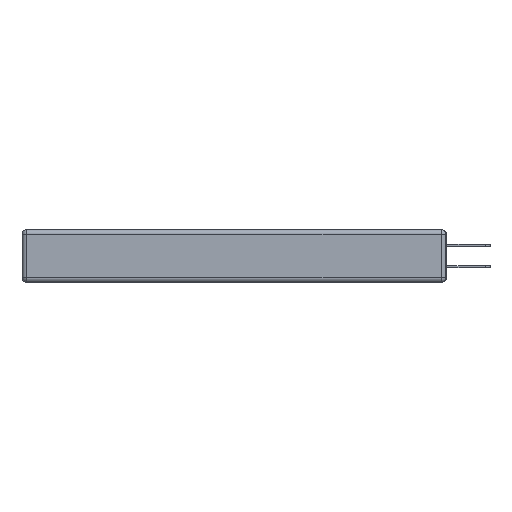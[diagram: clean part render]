
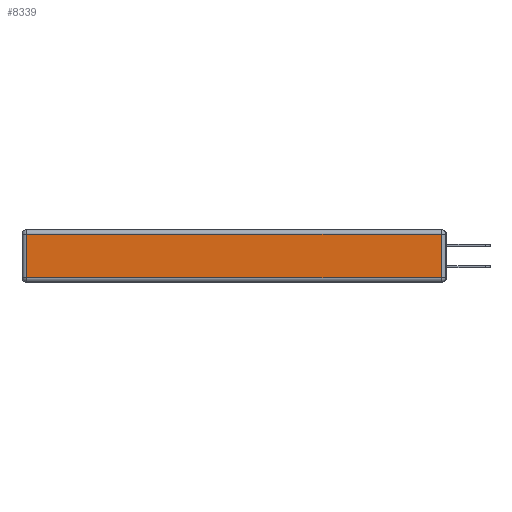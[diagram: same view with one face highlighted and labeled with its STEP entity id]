
A CAD part, left-side view. The second image highlights one B-rep face of the part: STEP entity #8339.
In plain terms, the highlighted planar face has unit normal (-1, 0, 0).
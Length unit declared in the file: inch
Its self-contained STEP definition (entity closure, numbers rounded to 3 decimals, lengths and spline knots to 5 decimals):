
#351 = LINE ( 'NONE', #5367, #19564 ) ;
#704 = LINE ( 'NONE', #6804, #16966 ) ;
#1762 = VECTOR ( 'NONE', #7961, 39.37008 ) ;
#1883 = VERTEX_POINT ( 'NONE', #20078 ) ;
#1894 = CARTESIAN_POINT ( 'NONE',  ( 0., 2.72, -0.343 ) ) ;
#1970 = EDGE_CURVE ( 'NONE', #1883, #16250, #351, .T. ) ;
#2259 = ORIENTED_EDGE ( 'NONE', *, *, #18672, .T. ) ;
#2781 = LINE ( 'NONE', #1894, #14357 ) ;
#3559 = VERTEX_POINT ( 'NONE', #10665 ) ;
#3735 = EDGE_CURVE ( 'NONE', #16250, #3559, #2781, .T. ) ;
#3833 = DIRECTION ( 'NONE',  ( 0., 0., 1. ) ) ;
#4417 = CARTESIAN_POINT ( 'NONE',  ( 0., 0., -0.343 ) ) ;
#5367 = CARTESIAN_POINT ( 'NONE',  ( 0., 2.75, -0.03 ) ) ;
#5632 = ORIENTED_EDGE ( 'NONE', *, *, #3735, .T. ) ;
#6016 = AXIS2_PLACEMENT_3D ( 'NONE', #4417, #10777, #7535 ) ;
#6289 = CARTESIAN_POINT ( 'NONE',  ( 0., 0., -0.313 ) ) ;
#6588 = CARTESIAN_POINT ( 'NONE',  ( 0., 2.72, -0.03 ) ) ;
#6804 = CARTESIAN_POINT ( 'NONE',  ( 0., 0.03, -0.343 ) ) ;
#6944 = ORIENTED_EDGE ( 'NONE', *, *, #1970, .T. ) ;
#7535 = DIRECTION ( 'NONE',  ( 0., 0., 1. ) ) ;
#7961 = DIRECTION ( 'NONE',  ( 0., -1., 0. ) ) ;
#8339 = ADVANCED_FACE ( 'NONE', ( #10236 ), #15301, .T. ) ;
#9081 = DIRECTION ( 'NONE',  ( 0., 1., 0. ) ) ;
#10236 = FACE_OUTER_BOUND ( 'NONE', #13064, .T. ) ;
#10665 = CARTESIAN_POINT ( 'NONE',  ( 0., 2.72, -0.313 ) ) ;
#10777 = DIRECTION ( 'NONE',  ( -1., 0., 0. ) ) ;
#10798 = ORIENTED_EDGE ( 'NONE', *, *, #13853, .T. ) ;
#11826 = VERTEX_POINT ( 'NONE', #14812 ) ;
#12769 = DIRECTION ( 'NONE',  ( 0., 0., -1. ) ) ;
#13064 = EDGE_LOOP ( 'NONE', ( #2259, #10798, #6944, #5632 ) ) ;
#13601 = LINE ( 'NONE', #6289, #1762 ) ;
#13853 = EDGE_CURVE ( 'NONE', #11826, #1883, #704, .T. ) ;
#14357 = VECTOR ( 'NONE', #12769, 39.37008 ) ;
#14812 = CARTESIAN_POINT ( 'NONE',  ( 0., 0.03, -0.313 ) ) ;
#15301 = PLANE ( 'NONE',  #6016 ) ;
#16250 = VERTEX_POINT ( 'NONE', #6588 ) ;
#16966 = VECTOR ( 'NONE', #3833, 39.37008 ) ;
#18672 = EDGE_CURVE ( 'NONE', #3559, #11826, #13601, .T. ) ;
#19564 = VECTOR ( 'NONE', #9081, 39.37008 ) ;
#20078 = CARTESIAN_POINT ( 'NONE',  ( 0., 0.03, -0.03 ) ) ;
